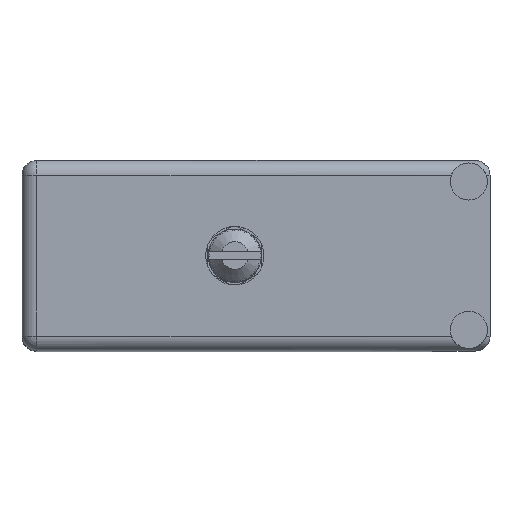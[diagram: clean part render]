
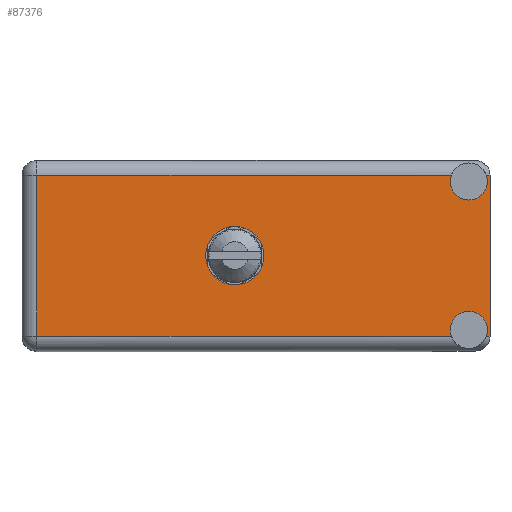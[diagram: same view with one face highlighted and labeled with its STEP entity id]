
A CAD part, top view. The second image highlights one B-rep face of the part: STEP entity #87376.
In plain terms, the highlighted face is planar.
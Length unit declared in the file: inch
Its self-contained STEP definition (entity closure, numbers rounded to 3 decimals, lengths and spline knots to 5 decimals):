
#978 = EDGE_CURVE ( 'NONE', #53339, #53403, #17535, .T. ) ;
#3807 = CIRCLE ( 'NONE', #34057, 0.0875 ) ;
#5351 = EDGE_CURVE ( 'NONE', #82439, #39933, #54308, .T. ) ;
#5435 = FACE_BOUND ( 'NONE', #67643, .T. ) ;
#5790 = CARTESIAN_POINT ( 'NONE',  ( 0.07, 1.566, -0.829 ) ) ;
#7084 = CARTESIAN_POINT ( 'NONE',  ( 2.208, 1.566, -0.07 ) ) ;
#7988 = CARTESIAN_POINT ( 'NONE',  ( 2.02562, 1.566, -0.07 ) ) ;
#8044 = ORIENTED_EDGE ( 'NONE', *, *, #56566, .F. ) ;
#8603 = ORIENTED_EDGE ( 'NONE', *, *, #75935, .F. ) ;
#10865 = DIRECTION ( 'NONE',  ( 0., 1., 0. ) ) ;
#11936 = EDGE_CURVE ( 'NONE', #17148, #53588, #80689, .T. ) ;
#13418 = ORIENTED_EDGE ( 'NONE', *, *, #72957, .F. ) ;
#14365 = CARTESIAN_POINT ( 'NONE',  ( 0.07, 1.566, -0.07 ) ) ;
#14368 = EDGE_LOOP ( 'NONE', ( #77292, #28023, #72203, #70260, #95151, #78162, #70789, #8044, #76529, #95686 ) ) ;
#16696 = DIRECTION ( 'NONE',  ( 0., 1., 0. ) ) ;
#17148 = VERTEX_POINT ( 'NONE', #102390 ) ;
#17535 = LINE ( 'NONE', #82305, #59650 ) ;
#18334 = DIRECTION ( 'NONE',  ( 0., 0., 1. ) ) ;
#22800 = DIRECTION ( 'NONE',  ( 0., 1., 0. ) ) ;
#23531 = CARTESIAN_POINT ( 'NONE',  ( 2.108, 1.566, -0.7995 ) ) ;
#23713 = CARTESIAN_POINT ( 'NONE',  ( 2.208, 1.566, -0.829 ) ) ;
#24901 = DIRECTION ( 'NONE',  ( 1., 0., 0. ) ) ;
#25104 = CARTESIAN_POINT ( 'NONE',  ( 0.07, 1.566, -0.899 ) ) ;
#25606 = CARTESIAN_POINT ( 'NONE',  ( 2.208, 1.566, -0.07 ) ) ;
#28023 = ORIENTED_EDGE ( 'NONE', *, *, #37132, .F. ) ;
#29329 = AXIS2_PLACEMENT_3D ( 'NONE', #96534, #49629, #97055 ) ;
#29642 = CARTESIAN_POINT ( 'NONE',  ( 1.004, 1.566, -0.4495 ) ) ;
#29867 = VECTOR ( 'NONE', #71744, 39.37008 ) ;
#32476 = VECTOR ( 'NONE', #65659, 39.37008 ) ;
#34057 = AXIS2_PLACEMENT_3D ( 'NONE', #88361, #16696, #87809 ) ;
#34225 = CIRCLE ( 'NONE', #59491, 0.1375 ) ;
#35512 = VERTEX_POINT ( 'NONE', #58890 ) ;
#36863 = CIRCLE ( 'NONE', #50319, 0.0875 ) ;
#37132 = EDGE_CURVE ( 'NONE', #46940, #53403, #89913, .T. ) ;
#37584 = FACE_OUTER_BOUND ( 'NONE', #14368, .T. ) ;
#38331 = LINE ( 'NONE', #25606, #32476 ) ;
#39142 = CARTESIAN_POINT ( 'NONE',  ( 0., 1.566, -0.899 ) ) ;
#39380 = LINE ( 'NONE', #25104, #99787 ) ;
#39933 = VERTEX_POINT ( 'NONE', #68978 ) ;
#42985 = EDGE_CURVE ( 'NONE', #102549, #64102, #38331, .T. ) ;
#42995 = DIRECTION ( 'NONE',  ( 0., 0., 1. ) ) ;
#43572 = DIRECTION ( 'NONE',  ( 0., 0., 1. ) ) ;
#44739 = EDGE_CURVE ( 'NONE', #53588, #53339, #39380, .T. ) ;
#46169 = AXIS2_PLACEMENT_3D ( 'NONE', #23531, #88889, #80445 ) ;
#46940 = VERTEX_POINT ( 'NONE', #56658 ) ;
#47168 = EDGE_CURVE ( 'NONE', #50728, #39933, #89942, .T. ) ;
#47436 = CARTESIAN_POINT ( 'NONE',  ( 0., 1.566, -0.829 ) ) ;
#48324 = DIRECTION ( 'NONE',  ( 0., 0., 1. ) ) ;
#49629 = DIRECTION ( 'NONE',  ( 0., 1., 0. ) ) ;
#50319 = AXIS2_PLACEMENT_3D ( 'NONE', #50470, #74731, #18334 ) ;
#50470 = CARTESIAN_POINT ( 'NONE',  ( 2.108, 1.566, -0.0995 ) ) ;
#50728 = VERTEX_POINT ( 'NONE', #56173 ) ;
#52066 = CARTESIAN_POINT ( 'NONE',  ( 2.19038, 1.566, -0.07 ) ) ;
#52869 = VERTEX_POINT ( 'NONE', #76794 ) ;
#53339 = VERTEX_POINT ( 'NONE', #14365 ) ;
#53403 = VERTEX_POINT ( 'NONE', #7988 ) ;
#53588 = VERTEX_POINT ( 'NONE', #5790 ) ;
#54308 = LINE ( 'NONE', #47436, #83680 ) ;
#54953 = DIRECTION ( 'NONE',  ( 0., 0., 1. ) ) ;
#55486 = VECTOR ( 'NONE', #43572, 39.37008 ) ;
#56173 = CARTESIAN_POINT ( 'NONE',  ( 2.108, 1.566, -0.712 ) ) ;
#56481 = CARTESIAN_POINT ( 'NONE',  ( 0., 1.566, -0.829 ) ) ;
#56566 = EDGE_CURVE ( 'NONE', #17148, #50728, #3807, .T. ) ;
#56658 = CARTESIAN_POINT ( 'NONE',  ( 2.108, 1.566, -0.187 ) ) ;
#58890 = CARTESIAN_POINT ( 'NONE',  ( 1.004, 1.566, -0.312 ) ) ;
#59491 = AXIS2_PLACEMENT_3D ( 'NONE', #29642, #100814, #92905 ) ;
#59650 = VECTOR ( 'NONE', #24901, 39.37008 ) ;
#64102 = VERTEX_POINT ( 'NONE', #7084 ) ;
#65659 = DIRECTION ( 'NONE',  ( 1., 0., 0. ) ) ;
#67643 = EDGE_LOOP ( 'NONE', ( #8603, #13418 ) ) ;
#68634 = EDGE_CURVE ( 'NONE', #102549, #46940, #36863, .T. ) ;
#68978 = CARTESIAN_POINT ( 'NONE',  ( 2.19038, 1.566, -0.829 ) ) ;
#70260 = ORIENTED_EDGE ( 'NONE', *, *, #42985, .T. ) ;
#70618 = DIRECTION ( 'NONE',  ( -1., 0., 0. ) ) ;
#70789 = ORIENTED_EDGE ( 'NONE', *, *, #47168, .F. ) ;
#71744 = DIRECTION ( 'NONE',  ( -1., 0., 0. ) ) ;
#72203 = ORIENTED_EDGE ( 'NONE', *, *, #68634, .F. ) ;
#72957 = EDGE_CURVE ( 'NONE', #52869, #35512, #103036, .T. ) ;
#74731 = DIRECTION ( 'NONE',  ( 0., 1., 0. ) ) ;
#75935 = EDGE_CURVE ( 'NONE', #35512, #52869, #34225, .T. ) ;
#76529 = ORIENTED_EDGE ( 'NONE', *, *, #11936, .T. ) ;
#76794 = CARTESIAN_POINT ( 'NONE',  ( 1.004, 1.566, -0.587 ) ) ;
#77207 = CARTESIAN_POINT ( 'NONE',  ( 1.004, 1.566, -0.4495 ) ) ;
#77292 = ORIENTED_EDGE ( 'NONE', *, *, #978, .T. ) ;
#77979 = EDGE_CURVE ( 'NONE', #82439, #64102, #97855, .T. ) ;
#78162 = ORIENTED_EDGE ( 'NONE', *, *, #5351, .T. ) ;
#80445 = DIRECTION ( 'NONE',  ( 0., 0., 1. ) ) ;
#80689 = LINE ( 'NONE', #56481, #29867 ) ;
#82305 = CARTESIAN_POINT ( 'NONE',  ( 2.208, 1.566, -0.07 ) ) ;
#82439 = VERTEX_POINT ( 'NONE', #23713 ) ;
#82898 = AXIS2_PLACEMENT_3D ( 'NONE', #77207, #10865, #42995 ) ;
#83680 = VECTOR ( 'NONE', #70618, 39.37008 ) ;
#87376 = ADVANCED_FACE ( 'NONE', ( #5435, #37584 ), #95005, .T. ) ;
#87809 = DIRECTION ( 'NONE',  ( 0., 0., 1. ) ) ;
#88361 = CARTESIAN_POINT ( 'NONE',  ( 2.108, 1.566, -0.7995 ) ) ;
#88889 = DIRECTION ( 'NONE',  ( 0., 1., 0. ) ) ;
#89913 = CIRCLE ( 'NONE', #29329, 0.0875 ) ;
#89942 = CIRCLE ( 'NONE', #46169, 0.0875 ) ;
#92905 = DIRECTION ( 'NONE',  ( 0., 0., 1. ) ) ;
#95005 = PLANE ( 'NONE',  #97142 ) ;
#95151 = ORIENTED_EDGE ( 'NONE', *, *, #77979, .F. ) ;
#95686 = ORIENTED_EDGE ( 'NONE', *, *, #44739, .T. ) ;
#96534 = CARTESIAN_POINT ( 'NONE',  ( 2.108, 1.566, -0.0995 ) ) ;
#97055 = DIRECTION ( 'NONE',  ( 0., 0., 1. ) ) ;
#97142 = AXIS2_PLACEMENT_3D ( 'NONE', #39142, #22800, #54953 ) ;
#97855 = LINE ( 'NONE', #98897, #55486 ) ;
#98897 = CARTESIAN_POINT ( 'NONE',  ( 2.208, 1.566, 0. ) ) ;
#99787 = VECTOR ( 'NONE', #48324, 39.37008 ) ;
#100814 = DIRECTION ( 'NONE',  ( 0., 1., 0. ) ) ;
#102390 = CARTESIAN_POINT ( 'NONE',  ( 2.02562, 1.566, -0.829 ) ) ;
#102549 = VERTEX_POINT ( 'NONE', #52066 ) ;
#103036 = CIRCLE ( 'NONE', #82898, 0.1375 ) ;
